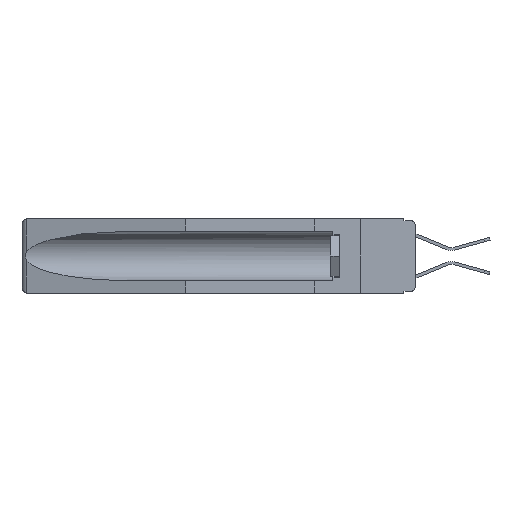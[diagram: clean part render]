
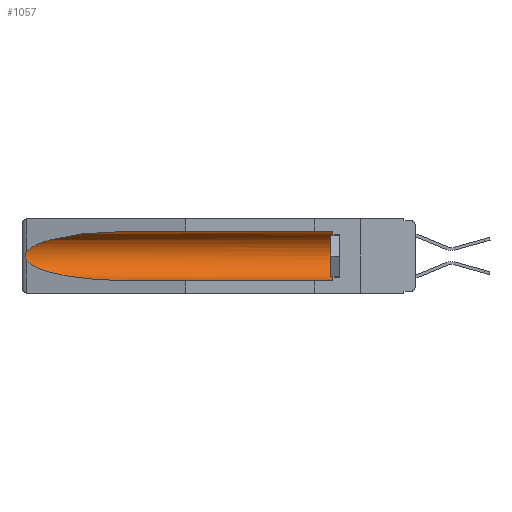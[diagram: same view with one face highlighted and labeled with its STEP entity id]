
A CAD part, left-side view. The second image highlights one B-rep face of the part: STEP entity #1057.
In plain terms, the highlighted cylindrical face has radius 2.857 mm (diameter 5.715 mm), a partial arc.
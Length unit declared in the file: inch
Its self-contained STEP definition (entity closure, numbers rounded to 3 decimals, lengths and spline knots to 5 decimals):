
#612 = CARTESIAN_POINT ( 'NONE',  ( 0.26537, 1.52718, -0.14972 ) ) ;
#635 = LINE ( 'NONE', #15491, #9573 ) ;
#1057 = ADVANCED_FACE ( 'NONE', ( #22368 ), #4404, .F. ) ;
#1099 = CARTESIAN_POINT ( 'NONE',  ( 0.25451, 1.48313, -0.09465 ) ) ;
#1330 = CARTESIAN_POINT ( 'NONE',  ( 0.26537, 1.52718, -0.19328 ) ) ;
#1539 = CARTESIAN_POINT ( 'NONE',  ( 0.155, 0.126, -0.059 ) ) ;
#1691 = EDGE_LOOP ( 'NONE', ( #11823, #15747, #17177, #3658, #3947, #3901 ) ) ;
#3155 = CARTESIAN_POINT ( 'NONE',  ( 0.2675, 1.53308, -0.16763 ) ) ;
#3265 = CARTESIAN_POINT ( 'NONE',  ( 0.2673, 1.53269, -0.17917 ) ) ;
#3377 = AXIS2_PLACEMENT_3D ( 'NONE', #22813, #6305, #13649 ) ;
#3658 = ORIENTED_EDGE ( 'NONE', *, *, #6421, .F. ) ;
#3830 = DIRECTION ( 'NONE',  ( 0., 1., 0. ) ) ;
#3901 = ORIENTED_EDGE ( 'NONE', *, *, #8602, .T. ) ;
#3947 = ORIENTED_EDGE ( 'NONE', *, *, #16201, .T. ) ;
#4043 = DIRECTION ( 'NONE',  ( 0., 0., 1. ) ) ;
#4286 = DIRECTION ( 'NONE',  ( 0., 1., 0. ) ) ;
#4404 = CYLINDRICAL_SURFACE ( 'NONE', #8666, 0.1125 ) ;
#4754 = CARTESIAN_POINT ( 'NONE',  ( 0.155, 1.07973, -0.284 ) ) ;
#4971 = CARTESIAN_POINT ( 'NONE',  ( 0.26654, 1.53092, -0.15636 ) ) ;
#5000 = VERTEX_POINT ( 'NONE', #1539 ) ;
#5203 = CARTESIAN_POINT ( 'NONE',  ( 0.26597, 1.52961, -0.15275 ) ) ;
#5621 = VERTEX_POINT ( 'NONE', #11154 ) ;
#5635 = LINE ( 'NONE', #22384, #11398 ) ;
#5655 = B_SPLINE_CURVE_WITH_KNOTS ( 'NONE', 3,
 ( #21467, #5203, #4971, #12321, #3155, #17872, #3265, #14480, #7021, #1330 ),
 .UNSPECIFIED., .F., .F.,
 ( 4, 2, 2, 2, 4 ),
 ( 0., 0.00029, 0.00058, 0.00087, 0.00117 ),
 .UNSPECIFIED. ) ;
#6305 = DIRECTION ( 'NONE',  ( 0., -1., 0. ) ) ;
#6421 = EDGE_CURVE ( 'NONE', #13152, #23561, #5635, .T. ) ;
#7021 = CARTESIAN_POINT ( 'NONE',  ( 0.26597, 1.5296, -0.19026 ) ) ;
#8034 = CARTESIAN_POINT ( 'NONE',  ( 0.155, -0.30754, -0.1715 ) ) ;
#8602 = EDGE_CURVE ( 'NONE', #5000, #11360, #635, .T. ) ;
#8666 = AXIS2_PLACEMENT_3D ( 'NONE', #8034, #4286, #4043 ) ;
#8915 = CARTESIAN_POINT ( 'NONE',  ( 0.155, 1.07973, -0.059 ) ) ;
#9573 = VECTOR ( 'NONE', #19458, 39.37008 ) ;
#10188 = CARTESIAN_POINT ( 'NONE',  ( 0.155, 1.07973, -0.284 ) ) ;
#10306 = CARTESIAN_POINT ( 'NONE',  ( 0.21114, 1.30732, -0.284 ) ) ;
#10329 = CARTESIAN_POINT ( 'NONE',  ( 0.26537, 1.52718, -0.19328 ) ) ;
#10424 = EDGE_CURVE ( 'NONE', #11360, #5621, #17802, .T. ) ;
#11154 = CARTESIAN_POINT ( 'NONE',  ( 0.26537, 1.52718, -0.14972 ) ) ;
#11360 = VERTEX_POINT ( 'NONE', #8915 ) ;
#11398 = VECTOR ( 'NONE', #3830, 39.37008 ) ;
#11823 = ORIENTED_EDGE ( 'NONE', *, *, #10424, .T. ) ;
#11837 = CARTESIAN_POINT ( 'NONE',  ( 0.21114, 1.30732, -0.059 ) ) ;
#11964 = CARTESIAN_POINT ( 'NONE',  ( 0.155, 1.07973, -0.059 ) ) ;
#12321 = CARTESIAN_POINT ( 'NONE',  ( 0.2673, 1.5327, -0.16383 ) ) ;
#13028 = EDGE_CURVE ( 'NONE', #18035, #23561, #16085, .T. ) ;
#13152 = VERTEX_POINT ( 'NONE', #18013 ) ;
#13649 = DIRECTION ( 'NONE',  ( 0., 0., 1. ) ) ;
#14480 = CARTESIAN_POINT ( 'NONE',  ( 0.26655, 1.53094, -0.18657 ) ) ;
#15491 = CARTESIAN_POINT ( 'NONE',  ( 0.155, -0.30754, -0.059 ) ) ;
#15747 = ORIENTED_EDGE ( 'NONE', *, *, #19172, .T. ) ;
#15860 = CARTESIAN_POINT ( 'NONE',  ( 0.25451, 1.48313, -0.24835 ) ) ;
#16085 =( BOUNDED_CURVE ( )  B_SPLINE_CURVE ( 3, ( #17540, #15860, #10306, #10188 ),
 .UNSPECIFIED., .F., .F. ) 
 B_SPLINE_CURVE_WITH_KNOTS ( ( 4, 4 ),
 ( 0.1948, 1.5708 ),
 .UNSPECIFIED. ) 
 CURVE ( )  GEOMETRIC_REPRESENTATION_ITEM ( )  RATIONAL_B_SPLINE_CURVE ( ( 1., 0.848, 0.848, 1. ) ) 
 REPRESENTATION_ITEM ( '' )  );
#16201 = EDGE_CURVE ( 'NONE', #13152, #5000, #16489, .T. ) ;
#16489 = CIRCLE ( 'NONE', #3377, 0.1125 ) ;
#17177 = ORIENTED_EDGE ( 'NONE', *, *, #13028, .T. ) ;
#17540 = CARTESIAN_POINT ( 'NONE',  ( 0.26537, 1.52718, -0.19328 ) ) ;
#17802 =( BOUNDED_CURVE ( )  B_SPLINE_CURVE ( 3, ( #11964, #11837, #1099, #612 ),
 .UNSPECIFIED., .F., .F. ) 
 B_SPLINE_CURVE_WITH_KNOTS ( ( 4, 4 ),
 ( 4.71239, 6.08839 ),
 .UNSPECIFIED. ) 
 CURVE ( )  GEOMETRIC_REPRESENTATION_ITEM ( )  RATIONAL_B_SPLINE_CURVE ( ( 1., 0.848, 0.848, 1. ) ) 
 REPRESENTATION_ITEM ( '' )  );
#17872 = CARTESIAN_POINT ( 'NONE',  ( 0.2675, 1.53308, -0.17534 ) ) ;
#18013 = CARTESIAN_POINT ( 'NONE',  ( 0.155, 0.126, -0.284 ) ) ;
#18035 = VERTEX_POINT ( 'NONE', #10329 ) ;
#19172 = EDGE_CURVE ( 'NONE', #5621, #18035, #5655, .T. ) ;
#19458 = DIRECTION ( 'NONE',  ( 0., 1., 0. ) ) ;
#21467 = CARTESIAN_POINT ( 'NONE',  ( 0.26537, 1.52718, -0.14972 ) ) ;
#22368 = FACE_OUTER_BOUND ( 'NONE', #1691, .T. ) ;
#22384 = CARTESIAN_POINT ( 'NONE',  ( 0.155, -0.30754, -0.284 ) ) ;
#22813 = CARTESIAN_POINT ( 'NONE',  ( 0.155, 0.126, -0.1715 ) ) ;
#23561 = VERTEX_POINT ( 'NONE', #4754 ) ;
